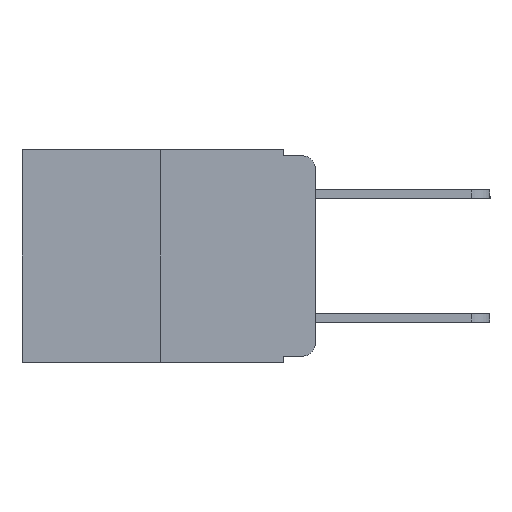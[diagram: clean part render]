
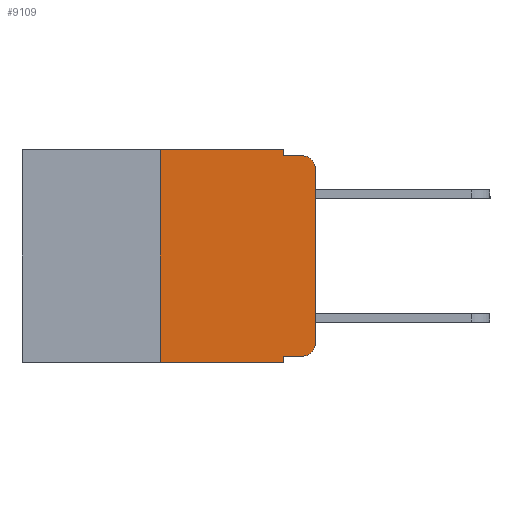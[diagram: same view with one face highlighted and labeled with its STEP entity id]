
A CAD part, left-side view. The second image highlights one B-rep face of the part: STEP entity #9109.
In plain terms, the highlighted planar face has unit normal (-1, 0, 0).
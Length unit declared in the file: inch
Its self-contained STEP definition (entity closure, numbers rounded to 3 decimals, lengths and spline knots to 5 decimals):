
#247 = PLANE ( 'NONE',  #11382 ) ;
#264 = VECTOR ( 'NONE', #19353, 39.37008 ) ;
#558 = CARTESIAN_POINT ( 'NONE',  ( 0., 0.473, -0.343 ) ) ;
#1150 = DIRECTION ( 'NONE',  ( 0., -1., 0. ) ) ;
#1164 = VERTEX_POINT ( 'NONE', #17517 ) ;
#1207 = CARTESIAN_POINT ( 'NONE',  ( 0., 0.25, -0.343 ) ) ;
#1295 = LINE ( 'NONE', #558, #18371 ) ;
#1525 = ORIENTED_EDGE ( 'NONE', *, *, #11334, .T. ) ;
#1548 = DIRECTION ( 'NONE',  ( 0., 0., 1. ) ) ;
#1576 = ORIENTED_EDGE ( 'NONE', *, *, #2215, .T. ) ;
#1866 = EDGE_CURVE ( 'NONE', #10296, #1164, #1295, .T. ) ;
#1885 = ORIENTED_EDGE ( 'NONE', *, *, #19564, .F. ) ;
#1938 = ORIENTED_EDGE ( 'NONE', *, *, #15302, .F. ) ;
#2050 = ORIENTED_EDGE ( 'NONE', *, *, #21993, .F. ) ;
#2075 = ORIENTED_EDGE ( 'NONE', *, *, #12103, .F. ) ;
#2134 = CARTESIAN_POINT ( 'NONE',  ( 0., 0.051, -0.01 ) ) ;
#2180 = DIRECTION ( 'NONE',  ( -1., 0., 0. ) ) ;
#2185 = ORIENTED_EDGE ( 'NONE', *, *, #1866, .T. ) ;
#2215 = EDGE_CURVE ( 'NONE', #5685, #3416, #12854, .T. ) ;
#2334 = ORIENTED_EDGE ( 'NONE', *, *, #11056, .F. ) ;
#2382 = ORIENTED_EDGE ( 'NONE', *, *, #18835, .T. ) ;
#2483 = DIRECTION ( 'NONE',  ( 0., 0., -1. ) ) ;
#2503 = VERTEX_POINT ( 'NONE', #15103 ) ;
#2637 = CARTESIAN_POINT ( 'NONE',  ( 0., 0.051, -0.01 ) ) ;
#2918 = AXIS2_PLACEMENT_3D ( 'NONE', #12639, #2180, #14232 ) ;
#2928 = ORIENTED_EDGE ( 'NONE', *, *, #13460, .T. ) ;
#2973 = VERTEX_POINT ( 'NONE', #13359 ) ;
#3416 = VERTEX_POINT ( 'NONE', #6589 ) ;
#4238 = DIRECTION ( 'NONE',  ( 1., 0., 0. ) ) ;
#4526 = CARTESIAN_POINT ( 'NONE',  ( 0., 0.051, -0.333 ) ) ;
#4636 = CARTESIAN_POINT ( 'NONE',  ( 0., 0.02, -0.333 ) ) ;
#5156 = VECTOR ( 'NONE', #16193, 39.37008 ) ;
#5171 = LINE ( 'NONE', #17954, #9864 ) ;
#5422 = VECTOR ( 'NONE', #1548, 39.37008 ) ;
#5685 = VERTEX_POINT ( 'NONE', #10263 ) ;
#5993 = LINE ( 'NONE', #10487, #5422 ) ;
#6178 = AXIS2_PLACEMENT_3D ( 'NONE', #9796, #20974, #11505 ) ;
#6589 = CARTESIAN_POINT ( 'NONE',  ( 0., 0.02, -0.01 ) ) ;
#7881 = CARTESIAN_POINT ( 'NONE',  ( 0., 0., -0.313 ) ) ;
#8371 = VERTEX_POINT ( 'NONE', #21784 ) ;
#8757 = EDGE_LOOP ( 'NONE', ( #1525, #1576, #1885, #1938, #2050, #2075, #2185, #2334, #2382, #2928 ) ) ;
#8906 = VECTOR ( 'NONE', #1150, 39.37008 ) ;
#9109 = ADVANCED_FACE ( 'NONE', ( #16509 ), #247, .F. ) ;
#9796 = CARTESIAN_POINT ( 'NONE',  ( 0., 0.02, -0.313 ) ) ;
#9864 = VECTOR ( 'NONE', #9960, 39.37008 ) ;
#9960 = DIRECTION ( 'NONE',  ( 0., 0., -1. ) ) ;
#10263 = CARTESIAN_POINT ( 'NONE',  ( 0., 0., -0.03 ) ) ;
#10296 = VERTEX_POINT ( 'NONE', #1207 ) ;
#10487 = CARTESIAN_POINT ( 'NONE',  ( 0., 0., 0. ) ) ;
#11048 = VERTEX_POINT ( 'NONE', #4636 ) ;
#11056 = EDGE_CURVE ( 'NONE', #8371, #1164, #5171, .T. ) ;
#11334 = EDGE_CURVE ( 'NONE', #16017, #5685, #5993, .T. ) ;
#11382 = AXIS2_PLACEMENT_3D ( 'NONE', #14363, #4238, #15993 ) ;
#11505 = DIRECTION ( 'NONE',  ( 0., 0., -1. ) ) ;
#11591 = VECTOR ( 'NONE', #2483, 39.37008 ) ;
#12103 = EDGE_CURVE ( 'NONE', #10296, #2973, #18855, .T. ) ;
#12639 = CARTESIAN_POINT ( 'NONE',  ( 0., 0.02, -0.03 ) ) ;
#12854 = CIRCLE ( 'NONE', #2918, 0.02 ) ;
#12879 = CARTESIAN_POINT ( 'NONE',  ( 0., 0.051, 0. ) ) ;
#13359 = CARTESIAN_POINT ( 'NONE',  ( 0., 0.25, 0. ) ) ;
#13460 = EDGE_CURVE ( 'NONE', #11048, #16017, #18842, .T. ) ;
#13693 = CARTESIAN_POINT ( 'NONE',  ( 0., 0.25, 0. ) ) ;
#13832 = LINE ( 'NONE', #2637, #264 ) ;
#14112 = LINE ( 'NONE', #4526, #5156 ) ;
#14232 = DIRECTION ( 'NONE',  ( 0., 0., -1. ) ) ;
#14363 = CARTESIAN_POINT ( 'NONE',  ( 0., 0.473, 0. ) ) ;
#14619 = VECTOR ( 'NONE', #16956, 39.37008 ) ;
#15103 = CARTESIAN_POINT ( 'NONE',  ( 0., 0.051, 0. ) ) ;
#15302 = EDGE_CURVE ( 'NONE', #2503, #19360, #20006, .T. ) ;
#15993 = DIRECTION ( 'NONE',  ( 0., 0., -1. ) ) ;
#16017 = VERTEX_POINT ( 'NONE', #7881 ) ;
#16193 = DIRECTION ( 'NONE',  ( 0., -1., 0. ) ) ;
#16226 = DIRECTION ( 'NONE',  ( 0., -1., 0. ) ) ;
#16509 = FACE_OUTER_BOUND ( 'NONE', #8757, .T. ) ;
#16956 = DIRECTION ( 'NONE',  ( 0., 0., 1. ) ) ;
#17517 = CARTESIAN_POINT ( 'NONE',  ( 0., 0.051, -0.343 ) ) ;
#17954 = CARTESIAN_POINT ( 'NONE',  ( 0., 0.051, 0. ) ) ;
#18371 = VECTOR ( 'NONE', #16226, 39.37008 ) ;
#18835 = EDGE_CURVE ( 'NONE', #8371, #11048, #14112, .T. ) ;
#18842 = CIRCLE ( 'NONE', #6178, 0.02 ) ;
#18855 = LINE ( 'NONE', #13693, #14619 ) ;
#19353 = DIRECTION ( 'NONE',  ( 0., -1., 0. ) ) ;
#19360 = VERTEX_POINT ( 'NONE', #2134 ) ;
#19564 = EDGE_CURVE ( 'NONE', #19360, #3416, #13832, .T. ) ;
#20006 = LINE ( 'NONE', #12879, #11591 ) ;
#20974 = DIRECTION ( 'NONE',  ( -1., 0., 0. ) ) ;
#21342 = CARTESIAN_POINT ( 'NONE',  ( 0., 0.473, 0. ) ) ;
#21695 = LINE ( 'NONE', #21342, #8906 ) ;
#21784 = CARTESIAN_POINT ( 'NONE',  ( 0., 0.051, -0.333 ) ) ;
#21993 = EDGE_CURVE ( 'NONE', #2973, #2503, #21695, .T. ) ;
